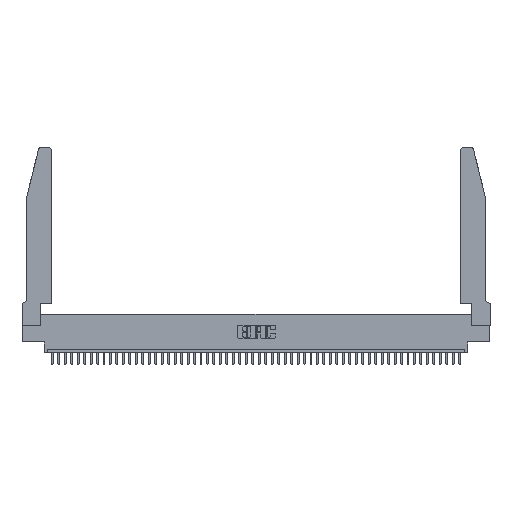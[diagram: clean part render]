
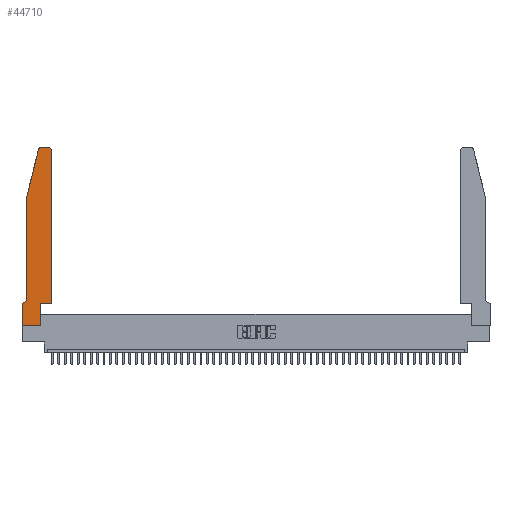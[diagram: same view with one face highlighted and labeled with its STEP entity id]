
A CAD part, top view. The second image highlights one B-rep face of the part: STEP entity #44710.
In plain terms, the highlighted planar face has unit normal (0, 0, 1).
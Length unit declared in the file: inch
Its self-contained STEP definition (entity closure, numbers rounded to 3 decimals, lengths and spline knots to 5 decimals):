
#690 = CARTESIAN_POINT ( 'NONE',  ( 0.0055, 0.42, 0.37 ) ) ;
#943 = CARTESIAN_POINT ( 'NONE',  ( 0.2865, 0., 0.37 ) ) ;
#1690 = EDGE_CURVE ( 'NONE', #36434, #21121, #1870, .T. ) ;
#1870 = LINE ( 'NONE', #5716, #36413 ) ;
#2604 = ORIENTED_EDGE ( 'NONE', *, *, #35900, .T. ) ;
#3089 = AXIS2_PLACEMENT_3D ( 'NONE', #36657, #28041, #4828 ) ;
#4004 = VECTOR ( 'NONE', #37640, 39.37008 ) ;
#4285 = VECTOR ( 'NONE', #27377, 39.37008 ) ;
#4512 = ORIENTED_EDGE ( 'NONE', *, *, #25371, .T. ) ;
#4670 = CARTESIAN_POINT ( 'NONE',  ( 0.4505, 0.35, 0.37 ) ) ;
#4828 = DIRECTION ( 'NONE',  ( 1., 0., 0. ) ) ;
#4871 = DIRECTION ( 'NONE',  ( 1., 0., 0. ) ) ;
#5716 = CARTESIAN_POINT ( 'NONE',  ( 0.0755, 0.35, 0.37 ) ) ;
#6076 = VECTOR ( 'NONE', #28703, 39.37008 ) ;
#7051 = VECTOR ( 'NONE', #18406, 39.37008 ) ;
#7935 = ORIENTED_EDGE ( 'NONE', *, *, #47574, .T. ) ;
#8532 = VECTOR ( 'NONE', #12025, 39.37008 ) ;
#8743 = CARTESIAN_POINT ( 'NONE',  ( 0., 0.35, 0.37 ) ) ;
#9657 = ORIENTED_EDGE ( 'NONE', *, *, #25969, .T. ) ;
#9732 = LINE ( 'NONE', #48493, #6076 ) ;
#10885 = ORIENTED_EDGE ( 'NONE', *, *, #29540, .T. ) ;
#11000 = ORIENTED_EDGE ( 'NONE', *, *, #1690, .T. ) ;
#12025 = DIRECTION ( 'NONE',  ( 0., -1., 0. ) ) ;
#12306 = DIRECTION ( 'NONE',  ( 1., 0., 0. ) ) ;
#12308 = CARTESIAN_POINT ( 'NONE',  ( 0.2865, 0.35, 0.37 ) ) ;
#13347 = EDGE_CURVE ( 'NONE', #21121, #24885, #28737, .T. ) ;
#15879 = LINE ( 'NONE', #44776, #24966 ) ;
#16687 = PLANE ( 'NONE',  #33651 ) ;
#17008 = LINE ( 'NONE', #23956, #4285 ) ;
#17020 = DIRECTION ( 'NONE',  ( 0., 0., 1. ) ) ;
#17200 = DIRECTION ( 'NONE',  ( 0., 1., 0. ) ) ;
#17397 = ORIENTED_EDGE ( 'NONE', *, *, #42562, .T. ) ;
#18406 = DIRECTION ( 'NONE',  ( -0.239, -0.971, 0. ) ) ;
#20147 = CARTESIAN_POINT ( 'NONE',  ( 0.0755, 2., 0.37 ) ) ;
#20538 = EDGE_CURVE ( 'NONE', #24885, #49704, #41387, .T. ) ;
#21001 = EDGE_CURVE ( 'NONE', #41085, #43699, #15879, .T. ) ;
#21121 = VERTEX_POINT ( 'NONE', #42242 ) ;
#23199 = CARTESIAN_POINT ( 'NONE',  ( 0., 0., 0.37 ) ) ;
#23790 = VECTOR ( 'NONE', #12306, 39.37008 ) ;
#23903 = EDGE_CURVE ( 'NONE', #39995, #47863, #28343, .T. ) ;
#23956 = CARTESIAN_POINT ( 'NONE',  ( 0.4505, 0.35, 0.37 ) ) ;
#24047 = DIRECTION ( 'NONE',  ( -1., 0., 0. ) ) ;
#24485 = DIRECTION ( 'NONE',  ( 0., 0., 1. ) ) ;
#24885 = VERTEX_POINT ( 'NONE', #23199 ) ;
#24966 = VECTOR ( 'NONE', #17200, 39.37008 ) ;
#25371 = EDGE_CURVE ( 'NONE', #47863, #46829, #46465, .T. ) ;
#25813 = LINE ( 'NONE', #36978, #4004 ) ;
#25969 = EDGE_CURVE ( 'NONE', #49704, #39010, #25813, .T. ) ;
#27235 = CARTESIAN_POINT ( 'NONE',  ( 0.0055, 0.35, 0.37 ) ) ;
#27377 = DIRECTION ( 'NONE',  ( 1., 0., 0. ) ) ;
#28041 = DIRECTION ( 'NONE',  ( 0., 0., 1. ) ) ;
#28343 = CIRCLE ( 'NONE', #3089, 0.03 ) ;
#28703 = DIRECTION ( 'NONE',  ( -1., 0., 0. ) ) ;
#28737 = LINE ( 'NONE', #37788, #48113 ) ;
#29152 = CARTESIAN_POINT ( 'NONE',  ( 0.284, 2.75, 0.37 ) ) ;
#29540 = EDGE_CURVE ( 'NONE', #43699, #48367, #45447, .T. ) ;
#29931 = CARTESIAN_POINT ( 'NONE',  ( 0.0755, 2., 0.37 ) ) ;
#31705 = DIRECTION ( 'NONE',  ( 0., 0., -1. ) ) ;
#32437 = AXIS2_PLACEMENT_3D ( 'NONE', #47185, #24485, #4871 ) ;
#33651 = AXIS2_PLACEMENT_3D ( 'NONE', #8743, #17020, #39706 ) ;
#33781 = CARTESIAN_POINT ( 'NONE',  ( 0.4505, 2.72, 0.37 ) ) ;
#34609 = CARTESIAN_POINT ( 'NONE',  ( 0.0755, 2., 0.37 ) ) ;
#35404 = EDGE_CURVE ( 'NONE', #48367, #39995, #9732, .T. ) ;
#35900 = EDGE_CURVE ( 'NONE', #36112, #36434, #37558, .T. ) ;
#36112 = VERTEX_POINT ( 'NONE', #48606 ) ;
#36263 = ORIENTED_EDGE ( 'NONE', *, *, #23903, .T. ) ;
#36413 = VECTOR ( 'NONE', #48557, 39.37008 ) ;
#36434 = VERTEX_POINT ( 'NONE', #27235 ) ;
#36657 = CARTESIAN_POINT ( 'NONE',  ( 0.284, 2.72, 0.37 ) ) ;
#36669 = ORIENTED_EDGE ( 'NONE', *, *, #35404, .T. ) ;
#36978 = CARTESIAN_POINT ( 'NONE',  ( 0.2865, 0.35, 0.37 ) ) ;
#37454 = DIRECTION ( 'NONE',  ( 0., -1., 0. ) ) ;
#37558 = CIRCLE ( 'NONE', #49594, 0.07 ) ;
#37640 = DIRECTION ( 'NONE',  ( 0., 1., 0. ) ) ;
#37788 = CARTESIAN_POINT ( 'NONE',  ( 0., 0., 0.37 ) ) ;
#38210 = LINE ( 'NONE', #20147, #8532 ) ;
#39010 = VERTEX_POINT ( 'NONE', #12308 ) ;
#39706 = DIRECTION ( 'NONE',  ( 1., 0., 0. ) ) ;
#39995 = VERTEX_POINT ( 'NONE', #29152 ) ;
#40123 = ORIENTED_EDGE ( 'NONE', *, *, #20538, .T. ) ;
#41085 = VERTEX_POINT ( 'NONE', #4670 ) ;
#41387 = LINE ( 'NONE', #43908, #23790 ) ;
#42242 = CARTESIAN_POINT ( 'NONE',  ( 0., 0.35, 0.37 ) ) ;
#42562 = EDGE_CURVE ( 'NONE', #46829, #36112, #38210, .T. ) ;
#43022 = CARTESIAN_POINT ( 'NONE',  ( 0.4205, 2.75, 0.37 ) ) ;
#43030 = ORIENTED_EDGE ( 'NONE', *, *, #21001, .T. ) ;
#43699 = VERTEX_POINT ( 'NONE', #33781 ) ;
#43908 = CARTESIAN_POINT ( 'NONE',  ( 0., 0., 0.37 ) ) ;
#44320 = ORIENTED_EDGE ( 'NONE', *, *, #13347, .T. ) ;
#44589 = FACE_OUTER_BOUND ( 'NONE', #45597, .T. ) ;
#44710 = ADVANCED_FACE ( 'NONE', ( #44589 ), #16687, .T. ) ;
#44776 = CARTESIAN_POINT ( 'NONE',  ( 0.4505, 0.35, 0.37 ) ) ;
#45447 = CIRCLE ( 'NONE', #32437, 0.03 ) ;
#45597 = EDGE_LOOP ( 'NONE', ( #36669, #36263, #4512, #17397, #2604, #11000, #44320, #40123, #9657, #7935, #43030, #10885 ) ) ;
#46465 = LINE ( 'NONE', #29931, #7051 ) ;
#46829 = VERTEX_POINT ( 'NONE', #34609 ) ;
#47185 = CARTESIAN_POINT ( 'NONE',  ( 0.4205, 2.72, 0.37 ) ) ;
#47574 = EDGE_CURVE ( 'NONE', #39010, #41085, #17008, .T. ) ;
#47863 = VERTEX_POINT ( 'NONE', #48506 ) ;
#48113 = VECTOR ( 'NONE', #37454, 39.37008 ) ;
#48367 = VERTEX_POINT ( 'NONE', #43022 ) ;
#48493 = CARTESIAN_POINT ( 'NONE',  ( 0.2605, 2.75, 0.37 ) ) ;
#48506 = CARTESIAN_POINT ( 'NONE',  ( 0.25487, 2.72718, 0.37 ) ) ;
#48557 = DIRECTION ( 'NONE',  ( -1., 0., 0. ) ) ;
#48606 = CARTESIAN_POINT ( 'NONE',  ( 0.0755, 0.42, 0.37 ) ) ;
#49594 = AXIS2_PLACEMENT_3D ( 'NONE', #690, #31705, #24047 ) ;
#49704 = VERTEX_POINT ( 'NONE', #943 ) ;
